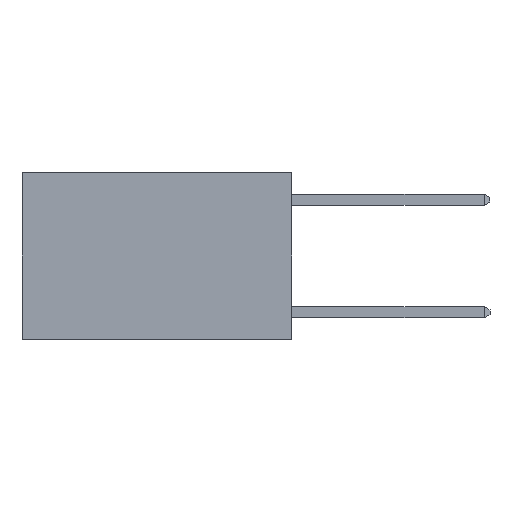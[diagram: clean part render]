
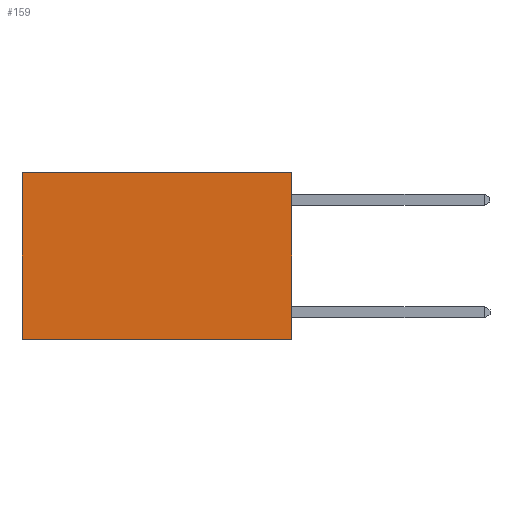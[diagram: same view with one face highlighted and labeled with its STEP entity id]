
A CAD part, left-side view. The second image highlights one B-rep face of the part: STEP entity #159.
In plain terms, the highlighted planar face has unit normal (-1, 0, 0).
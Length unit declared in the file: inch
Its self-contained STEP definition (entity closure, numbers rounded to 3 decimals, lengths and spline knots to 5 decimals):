
#83 = LINE ( 'NONE', #9050, #4072 ) ;
#159 = ADVANCED_FACE ( 'NONE', ( #5128 ), #2841, .F. ) ;
#863 = VECTOR ( 'NONE', #3307, 39.37008 ) ;
#947 = EDGE_CURVE ( 'NONE', #7530, #1142, #6395, .T. ) ;
#1097 = EDGE_CURVE ( 'NONE', #1142, #4522, #2987, .T. ) ;
#1142 = VERTEX_POINT ( 'NONE', #2714 ) ;
#1345 = ORIENTED_EDGE ( 'NONE', *, *, #1097, .F. ) ;
#1413 = VERTEX_POINT ( 'NONE', #8220 ) ;
#1607 = ORIENTED_EDGE ( 'NONE', *, *, #947, .F. ) ;
#2554 = LINE ( 'NONE', #3790, #8682 ) ;
#2681 = DIRECTION ( 'NONE',  ( 0., 0., -1. ) ) ;
#2714 = CARTESIAN_POINT ( 'NONE',  ( 0.2625, 0., -0.37 ) ) ;
#2841 = PLANE ( 'NONE',  #9173 ) ;
#2987 = LINE ( 'NONE', #3927, #863 ) ;
#3307 = DIRECTION ( 'NONE',  ( 0., 1., 0. ) ) ;
#3475 = EDGE_CURVE ( 'NONE', #1413, #4522, #2554, .T. ) ;
#3536 = CARTESIAN_POINT ( 'NONE',  ( 0.2625, 0., 0. ) ) ;
#3790 = CARTESIAN_POINT ( 'NONE',  ( 0.2625, 0.6, 0. ) ) ;
#3927 = CARTESIAN_POINT ( 'NONE',  ( 0.2625, 0., -0.37 ) ) ;
#3971 = ORIENTED_EDGE ( 'NONE', *, *, #4404, .T. ) ;
#4072 = VECTOR ( 'NONE', #9811, 39.37008 ) ;
#4230 = VECTOR ( 'NONE', #7045, 39.37008 ) ;
#4404 = EDGE_CURVE ( 'NONE', #7530, #1413, #83, .T. ) ;
#4445 = CARTESIAN_POINT ( 'NONE',  ( 0.2625, 0., 0. ) ) ;
#4522 = VERTEX_POINT ( 'NONE', #6826 ) ;
#4580 = DIRECTION ( 'NONE',  ( 0., 0., -1. ) ) ;
#5128 = FACE_OUTER_BOUND ( 'NONE', #5346, .T. ) ;
#5346 = EDGE_LOOP ( 'NONE', ( #7508, #1345, #1607, #3971 ) ) ;
#6395 = LINE ( 'NONE', #7546, #4230 ) ;
#6826 = CARTESIAN_POINT ( 'NONE',  ( 0.2625, 0.6, -0.37 ) ) ;
#7045 = DIRECTION ( 'NONE',  ( 0., 0., -1. ) ) ;
#7508 = ORIENTED_EDGE ( 'NONE', *, *, #3475, .T. ) ;
#7530 = VERTEX_POINT ( 'NONE', #3536 ) ;
#7546 = CARTESIAN_POINT ( 'NONE',  ( 0.2625, 0., 0. ) ) ;
#7917 = DIRECTION ( 'NONE',  ( 1., 0., 0. ) ) ;
#8220 = CARTESIAN_POINT ( 'NONE',  ( 0.2625, 0.6, 0. ) ) ;
#8682 = VECTOR ( 'NONE', #4580, 39.37008 ) ;
#9050 = CARTESIAN_POINT ( 'NONE',  ( 0.2625, 0., 0. ) ) ;
#9173 = AXIS2_PLACEMENT_3D ( 'NONE', #4445, #7917, #2681 ) ;
#9811 = DIRECTION ( 'NONE',  ( 0., 1., 0. ) ) ;
